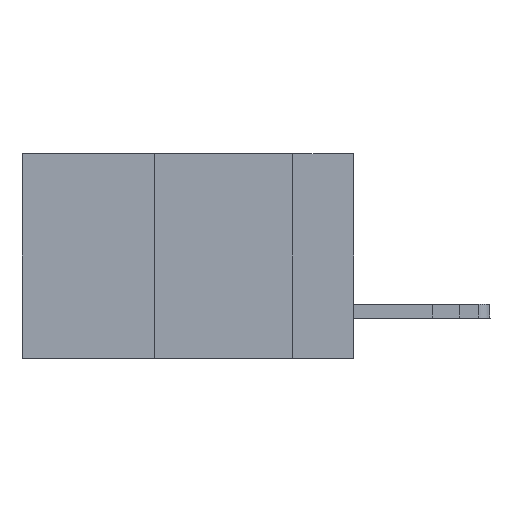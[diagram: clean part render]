
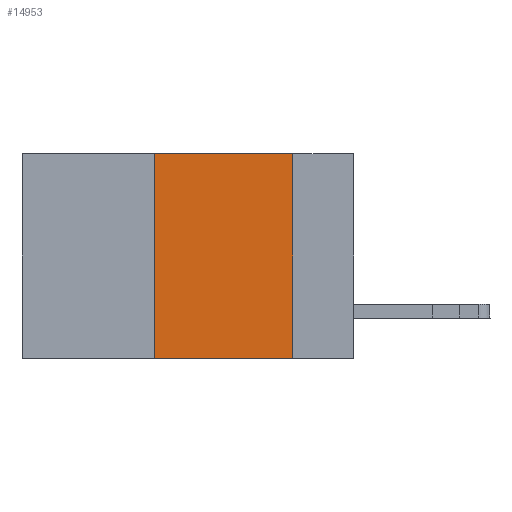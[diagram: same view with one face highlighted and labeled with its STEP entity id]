
A CAD part, left-side view. The second image highlights one B-rep face of the part: STEP entity #14953.
In plain terms, the highlighted planar face has unit normal (-1, 0, 0).
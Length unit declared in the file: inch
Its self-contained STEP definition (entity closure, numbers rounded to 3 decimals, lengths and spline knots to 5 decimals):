
#1131 = LINE ( 'NONE', #8506, #3759 ) ;
#1247 = EDGE_CURVE ( 'NONE', #2826, #15405, #10951, .T. ) ;
#1277 = PLANE ( 'NONE',  #12107 ) ;
#2826 = VERTEX_POINT ( 'NONE', #6012 ) ;
#3304 = CARTESIAN_POINT ( 'NONE',  ( 0., 0.36, 0. ) ) ;
#3759 = VECTOR ( 'NONE', #15845, 39.37008 ) ;
#3781 = VECTOR ( 'NONE', #12045, 39.37008 ) ;
#4302 = VECTOR ( 'NONE', #9533, 39.37008 ) ;
#4874 = CARTESIAN_POINT ( 'NONE',  ( 0., 0.11, -0.37 ) ) ;
#5177 = CARTESIAN_POINT ( 'NONE',  ( 0., 0.6, 0. ) ) ;
#5180 = ORIENTED_EDGE ( 'NONE', *, *, #14729, .F. ) ;
#6012 = CARTESIAN_POINT ( 'NONE',  ( 0., 0.36, -0.37 ) ) ;
#6419 = DIRECTION ( 'NONE',  ( 0., 0., -1. ) ) ;
#6500 = FACE_OUTER_BOUND ( 'NONE', #16145, .T. ) ;
#6543 = DIRECTION ( 'NONE',  ( 0., 0., -1. ) ) ;
#7613 = ORIENTED_EDGE ( 'NONE', *, *, #16161, .F. ) ;
#8019 = VECTOR ( 'NONE', #6543, 39.37008 ) ;
#8506 = CARTESIAN_POINT ( 'NONE',  ( 0., 0.6, 0. ) ) ;
#9087 = EDGE_CURVE ( 'NONE', #2826, #11255, #13319, .T. ) ;
#9533 = DIRECTION ( 'NONE',  ( 0., -1., 0. ) ) ;
#10118 = LINE ( 'NONE', #13958, #8019 ) ;
#10199 = CARTESIAN_POINT ( 'NONE',  ( 0., 0.36, 0. ) ) ;
#10360 = CARTESIAN_POINT ( 'NONE',  ( 0., 0.11, 0. ) ) ;
#10951 = LINE ( 'NONE', #14562, #4302 ) ;
#11255 = VERTEX_POINT ( 'NONE', #10199 ) ;
#12045 = DIRECTION ( 'NONE',  ( 0., 0., 1. ) ) ;
#12107 = AXIS2_PLACEMENT_3D ( 'NONE', #5177, #13839, #6419 ) ;
#12839 = ORIENTED_EDGE ( 'NONE', *, *, #1247, .T. ) ;
#13319 = LINE ( 'NONE', #3304, #3781 ) ;
#13839 = DIRECTION ( 'NONE',  ( 1., 0., 0. ) ) ;
#13958 = CARTESIAN_POINT ( 'NONE',  ( 0., 0.11, 0. ) ) ;
#13980 = VERTEX_POINT ( 'NONE', #10360 ) ;
#14490 = ORIENTED_EDGE ( 'NONE', *, *, #9087, .F. ) ;
#14562 = CARTESIAN_POINT ( 'NONE',  ( 0., 0.6, -0.37 ) ) ;
#14729 = EDGE_CURVE ( 'NONE', #11255, #13980, #1131, .T. ) ;
#14953 = ADVANCED_FACE ( 'NONE', ( #6500 ), #1277, .F. ) ;
#15405 = VERTEX_POINT ( 'NONE', #4874 ) ;
#15845 = DIRECTION ( 'NONE',  ( 0., -1., 0. ) ) ;
#16145 = EDGE_LOOP ( 'NONE', ( #7613, #5180, #14490, #12839 ) ) ;
#16161 = EDGE_CURVE ( 'NONE', #13980, #15405, #10118, .T. ) ;
